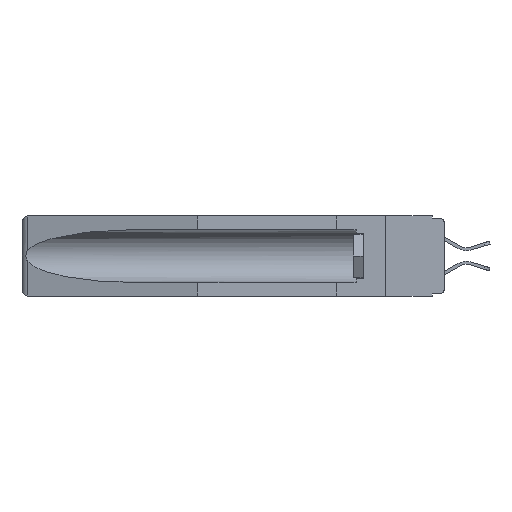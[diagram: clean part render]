
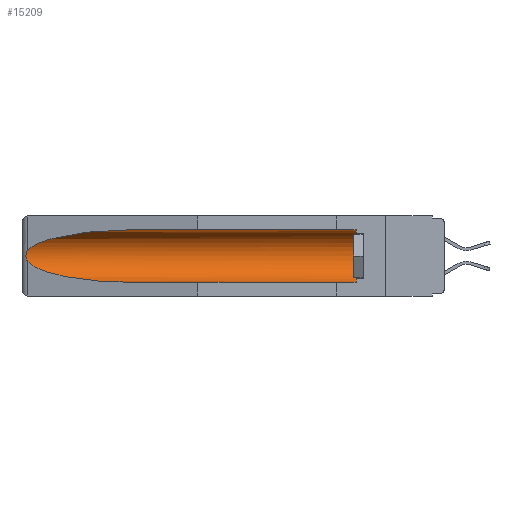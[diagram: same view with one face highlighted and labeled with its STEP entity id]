
A CAD part, left-side view. The second image highlights one B-rep face of the part: STEP entity #15209.
In plain terms, the highlighted cylindrical face has radius 2.857 mm (diameter 5.715 mm), a partial arc.
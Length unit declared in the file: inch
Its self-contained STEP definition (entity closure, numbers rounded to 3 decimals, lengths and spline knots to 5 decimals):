
#27 = ORIENTED_EDGE ( 'NONE', *, *, #13395, .F. ) ;
#170 = CARTESIAN_POINT ( 'NONE',  ( 0.155, -0.30754, -0.1715 ) ) ;
#779 = CARTESIAN_POINT ( 'NONE',  ( 0.25451, 1.48313, -0.24835 ) ) ;
#1231 = DIRECTION ( 'NONE',  ( 0., 1., 0. ) ) ;
#1363 = CARTESIAN_POINT ( 'NONE',  ( 0.155, 0.126, -0.284 ) ) ;
#1401 = DIRECTION ( 'NONE',  ( 0., 0., 1. ) ) ;
#1697 = CARTESIAN_POINT ( 'NONE',  ( 0.25451, 1.48313, -0.09465 ) ) ;
#1780 = ORIENTED_EDGE ( 'NONE', *, *, #8018, .T. ) ;
#1815 =( BOUNDED_CURVE ( )  B_SPLINE_CURVE ( 3, ( #8256, #5812, #1697, #1817 ),
 .UNSPECIFIED., .F., .F. ) 
 B_SPLINE_CURVE_WITH_KNOTS ( ( 4, 4 ),
 ( 4.71239, 6.08839 ),
 .UNSPECIFIED. ) 
 CURVE ( )  GEOMETRIC_REPRESENTATION_ITEM ( )  RATIONAL_B_SPLINE_CURVE ( ( 1., 0.848, 0.848, 1. ) ) 
 REPRESENTATION_ITEM ( '' )  );
#1817 = CARTESIAN_POINT ( 'NONE',  ( 0.26537, 1.52718, -0.14972 ) ) ;
#1823 = DIRECTION ( 'NONE',  ( 0., -1., 0. ) ) ;
#2136 = CIRCLE ( 'NONE', #12677, 0.1125 ) ;
#2567 = CARTESIAN_POINT ( 'NONE',  ( 0.155, 0.126, -0.059 ) ) ;
#3582 = CARTESIAN_POINT ( 'NONE',  ( 0.26597, 1.52961, -0.15275 ) ) ;
#3591 =( BOUNDED_CURVE ( )  B_SPLINE_CURVE ( 3, ( #12532, #779, #12648, #16431 ),
 .UNSPECIFIED., .F., .T. ) 
 B_SPLINE_CURVE_WITH_KNOTS ( ( 4, 4 ),
 ( 0.1948, 1.5708 ),
 .UNSPECIFIED. ) 
 CURVE ( )  GEOMETRIC_REPRESENTATION_ITEM ( )  RATIONAL_B_SPLINE_CURVE ( ( 1., 0.848, 0.848, 1. ) ) 
 REPRESENTATION_ITEM ( '' )  );
#3807 = DIRECTION ( 'NONE',  ( 0., 1., 0. ) ) ;
#3813 = CARTESIAN_POINT ( 'NONE',  ( 0.2675, 1.53308, -0.17534 ) ) ;
#4698 = EDGE_CURVE ( 'NONE', #16350, #13724, #3591, .T. ) ;
#4806 = LINE ( 'NONE', #5656, #5026 ) ;
#5016 = CARTESIAN_POINT ( 'NONE',  ( 0.26537, 1.52718, -0.19328 ) ) ;
#5026 = VECTOR ( 'NONE', #12173, 39.37008 ) ;
#5122 = CARTESIAN_POINT ( 'NONE',  ( 0.26597, 1.5296, -0.19026 ) ) ;
#5536 = ORIENTED_EDGE ( 'NONE', *, *, #9275, .T. ) ;
#5656 = CARTESIAN_POINT ( 'NONE',  ( 0.155, -0.30754, -0.284 ) ) ;
#5812 = CARTESIAN_POINT ( 'NONE',  ( 0.21114, 1.30732, -0.059 ) ) ;
#6035 = ORIENTED_EDGE ( 'NONE', *, *, #4698, .T. ) ;
#6115 = CARTESIAN_POINT ( 'NONE',  ( 0.26537, 1.52718, -0.19328 ) ) ;
#6298 = VERTEX_POINT ( 'NONE', #1363 ) ;
#6758 = EDGE_CURVE ( 'NONE', #13063, #11513, #1815, .T. ) ;
#6950 = EDGE_CURVE ( 'NONE', #14810, #13063, #7004, .T. ) ;
#6975 = FACE_OUTER_BOUND ( 'NONE', #9335, .T. ) ;
#7004 = LINE ( 'NONE', #7548, #16056 ) ;
#7548 = CARTESIAN_POINT ( 'NONE',  ( 0.155, -0.30754, -0.059 ) ) ;
#7738 = CARTESIAN_POINT ( 'NONE',  ( 0.2673, 1.53269, -0.17917 ) ) ;
#8018 = EDGE_CURVE ( 'NONE', #6298, #14810, #2136, .T. ) ;
#8206 = CARTESIAN_POINT ( 'NONE',  ( 0.155, 0.126, -0.1715 ) ) ;
#8256 = CARTESIAN_POINT ( 'NONE',  ( 0.155, 1.07973, -0.059 ) ) ;
#8401 = CYLINDRICAL_SURFACE ( 'NONE', #16833, 0.1125 ) ;
#8617 = CARTESIAN_POINT ( 'NONE',  ( 0.26537, 1.52718, -0.14972 ) ) ;
#8870 = CARTESIAN_POINT ( 'NONE',  ( 0.26654, 1.53092, -0.15636 ) ) ;
#8872 = CARTESIAN_POINT ( 'NONE',  ( 0.155, 1.07973, -0.284 ) ) ;
#9275 = EDGE_CURVE ( 'NONE', #11513, #16350, #10707, .T. ) ;
#9335 = EDGE_LOOP ( 'NONE', ( #14478, #5536, #6035, #27, #1780, #11592 ) ) ;
#10707 = B_SPLINE_CURVE_WITH_KNOTS ( 'NONE', 3,
 ( #12844, #3582, #8870, #11645, #14211, #3813, #7738, #12956, #5122, #5016 ),
 .UNSPECIFIED., .F., .F.,
 ( 4, 2, 2, 2, 4 ),
 ( 0., 0.00029, 0.00058, 0.00087, 0.00117 ),
 .UNSPECIFIED. ) ;
#10733 = DIRECTION ( 'NONE',  ( 0., 0., 1. ) ) ;
#11513 = VERTEX_POINT ( 'NONE', #8617 ) ;
#11592 = ORIENTED_EDGE ( 'NONE', *, *, #6950, .T. ) ;
#11645 = CARTESIAN_POINT ( 'NONE',  ( 0.2673, 1.5327, -0.16383 ) ) ;
#12173 = DIRECTION ( 'NONE',  ( 0., 1., 0. ) ) ;
#12532 = CARTESIAN_POINT ( 'NONE',  ( 0.26537, 1.52718, -0.19328 ) ) ;
#12648 = CARTESIAN_POINT ( 'NONE',  ( 0.21114, 1.30732, -0.284 ) ) ;
#12677 = AXIS2_PLACEMENT_3D ( 'NONE', #8206, #1823, #10733 ) ;
#12844 = CARTESIAN_POINT ( 'NONE',  ( 0.26537, 1.52718, -0.14972 ) ) ;
#12956 = CARTESIAN_POINT ( 'NONE',  ( 0.26655, 1.53094, -0.18657 ) ) ;
#13063 = VERTEX_POINT ( 'NONE', #16711 ) ;
#13395 = EDGE_CURVE ( 'NONE', #6298, #13724, #4806, .T. ) ;
#13724 = VERTEX_POINT ( 'NONE', #8872 ) ;
#14211 = CARTESIAN_POINT ( 'NONE',  ( 0.2675, 1.53308, -0.16763 ) ) ;
#14478 = ORIENTED_EDGE ( 'NONE', *, *, #6758, .T. ) ;
#14810 = VERTEX_POINT ( 'NONE', #2567 ) ;
#15209 = ADVANCED_FACE ( 'NONE', ( #6975 ), #8401, .F. ) ;
#16056 = VECTOR ( 'NONE', #3807, 39.37008 ) ;
#16350 = VERTEX_POINT ( 'NONE', #6115 ) ;
#16431 = CARTESIAN_POINT ( 'NONE',  ( 0.155, 1.07973, -0.284 ) ) ;
#16711 = CARTESIAN_POINT ( 'NONE',  ( 0.155, 1.07973, -0.059 ) ) ;
#16833 = AXIS2_PLACEMENT_3D ( 'NONE', #170, #1231, #1401 ) ;
